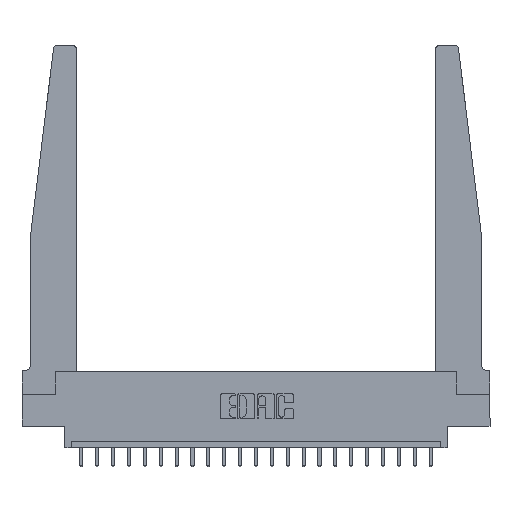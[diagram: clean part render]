
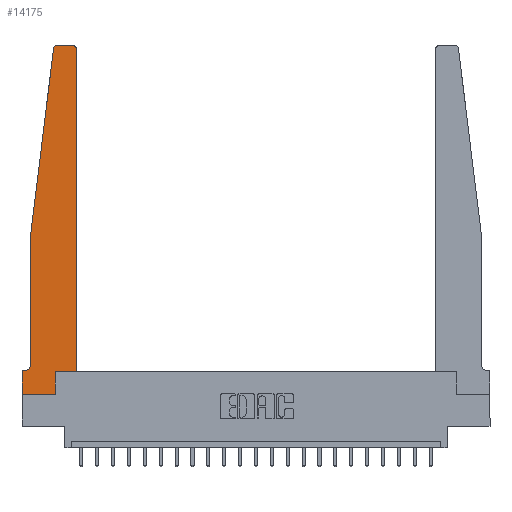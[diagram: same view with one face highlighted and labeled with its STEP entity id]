
A CAD part, top view. The second image highlights one B-rep face of the part: STEP entity #14175.
In plain terms, the highlighted planar face has unit normal (0, 0, 1).
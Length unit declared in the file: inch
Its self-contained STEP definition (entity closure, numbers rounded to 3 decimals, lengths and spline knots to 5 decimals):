
#63 = CARTESIAN_POINT ( 'NONE',  ( 0.425, 2.72, 0.37 ) ) ;
#163 = CARTESIAN_POINT ( 'NONE',  ( 0.065, 1.25, 0.37 ) ) ;
#206 = LINE ( 'NONE', #10738, #3052 ) ;
#305 = CARTESIAN_POINT ( 'NONE',  ( 0.2605, 0.18, 0.37 ) ) ;
#558 = EDGE_CURVE ( 'NONE', #3870, #2490, #2287, .T. ) ;
#1095 = EDGE_CURVE ( 'NONE', #10275, #9948, #206, .T. ) ;
#1131 = CARTESIAN_POINT ( 'NONE',  ( 0.25, 2.75, 0.37 ) ) ;
#1744 = VERTEX_POINT ( 'NONE', #19078 ) ;
#1785 = EDGE_CURVE ( 'NONE', #5472, #21026, #10588, .T. ) ;
#1889 = CARTESIAN_POINT ( 'NONE',  ( 0.27653, 2.75, 0.37 ) ) ;
#2123 = CARTESIAN_POINT ( 'NONE',  ( 0.2605, 0., 0.37 ) ) ;
#2154 = CARTESIAN_POINT ( 'NONE',  ( 0.065, 1.25, 0.37 ) ) ;
#2287 = CIRCLE ( 'NONE', #14850, 0.03 ) ;
#2384 = VERTEX_POINT ( 'NONE', #19950 ) ;
#2490 = VERTEX_POINT ( 'NONE', #11641 ) ;
#2630 = PLANE ( 'NONE',  #18287 ) ;
#2847 = LINE ( 'NONE', #16521, #13620 ) ;
#3021 = CARTESIAN_POINT ( 'NONE',  ( 0., 0., 0.37 ) ) ;
#3052 = VECTOR ( 'NONE', #17591, 39.37008 ) ;
#3132 = DIRECTION ( 'NONE',  ( 0., -1., 0. ) ) ;
#3254 = EDGE_CURVE ( 'NONE', #21026, #3870, #16509, .T. ) ;
#3502 = ORIENTED_EDGE ( 'NONE', *, *, #3254, .T. ) ;
#3577 = ORIENTED_EDGE ( 'NONE', *, *, #558, .T. ) ;
#3870 = VERTEX_POINT ( 'NONE', #1889 ) ;
#3942 = DIRECTION ( 'NONE',  ( 0., 0., -1. ) ) ;
#3983 = ORIENTED_EDGE ( 'NONE', *, *, #14107, .T. ) ;
#4412 = DIRECTION ( 'NONE',  ( 1., 0., 0. ) ) ;
#4774 = LINE ( 'NONE', #9807, #9773 ) ;
#4810 = LINE ( 'NONE', #3021, #7816 ) ;
#5472 = VERTEX_POINT ( 'NONE', #63 ) ;
#5702 = ORIENTED_EDGE ( 'NONE', *, *, #1785, .T. ) ;
#5886 = VECTOR ( 'NONE', #15826, 39.37008 ) ;
#6637 = CARTESIAN_POINT ( 'NONE',  ( 0.27653, 2.72, 0.37 ) ) ;
#6895 = LINE ( 'NONE', #163, #11553 ) ;
#7156 = ORIENTED_EDGE ( 'NONE', *, *, #13404, .T. ) ;
#7300 = ORIENTED_EDGE ( 'NONE', *, *, #17331, .T. ) ;
#7816 = VECTOR ( 'NONE', #3132, 39.37008 ) ;
#8459 = EDGE_CURVE ( 'NONE', #20569, #18451, #15411, .T. ) ;
#9541 = DIRECTION ( 'NONE',  ( -1., 0., 0. ) ) ;
#9643 = CARTESIAN_POINT ( 'NONE',  ( 0.065, 1.25, 0.37 ) ) ;
#9705 = CARTESIAN_POINT ( 'NONE',  ( 0.2605, 0.18, 0.37 ) ) ;
#9773 = VECTOR ( 'NONE', #18234, 39.37008 ) ;
#9807 = CARTESIAN_POINT ( 'NONE',  ( 0.065, 0.1875, 0.37 ) ) ;
#9948 = VERTEX_POINT ( 'NONE', #2123 ) ;
#10039 = AXIS2_PLACEMENT_3D ( 'NONE', #19746, #3942, #10870 ) ;
#10247 = EDGE_CURVE ( 'NONE', #2384, #10275, #4810, .T. ) ;
#10275 = VERTEX_POINT ( 'NONE', #20831 ) ;
#10371 = ORIENTED_EDGE ( 'NONE', *, *, #10247, .T. ) ;
#10466 = CARTESIAN_POINT ( 'NONE',  ( 0.065, 0.2375, 0.37 ) ) ;
#10588 = CIRCLE ( 'NONE', #19914, 0.03 ) ;
#10738 = CARTESIAN_POINT ( 'NONE',  ( 0., 0., 0.37 ) ) ;
#10870 = DIRECTION ( 'NONE',  ( -1., 0., 0. ) ) ;
#11105 = CARTESIAN_POINT ( 'NONE',  ( 0.395, 2.75, 0.37 ) ) ;
#11179 = DIRECTION ( 'NONE',  ( 1., 0., 0. ) ) ;
#11288 = CARTESIAN_POINT ( 'NONE',  ( 0.425, 0.18, 0.37 ) ) ;
#11553 = VECTOR ( 'NONE', #20481, 39.37008 ) ;
#11641 = CARTESIAN_POINT ( 'NONE',  ( 0.24675, 2.72367, 0.37 ) ) ;
#11917 = EDGE_CURVE ( 'NONE', #9948, #18796, #15677, .T. ) ;
#12160 = EDGE_LOOP ( 'NONE', ( #3502, #3577, #14645, #19969, #12771, #7300, #10371, #12710, #17135, #7156, #3983, #5702 ) ) ;
#12565 = DIRECTION ( 'NONE',  ( 1., 0., 0. ) ) ;
#12710 = ORIENTED_EDGE ( 'NONE', *, *, #1095, .T. ) ;
#12771 = ORIENTED_EDGE ( 'NONE', *, *, #8459, .T. ) ;
#13404 = EDGE_CURVE ( 'NONE', #18796, #1744, #20050, .T. ) ;
#13620 = VECTOR ( 'NONE', #19663, 39.37008 ) ;
#14107 = EDGE_CURVE ( 'NONE', #1744, #5472, #2847, .T. ) ;
#14175 = ADVANCED_FACE ( 'NONE', ( #16411 ), #2630, .T. ) ;
#14608 = CARTESIAN_POINT ( 'NONE',  ( 0., 0.1875, 0.37 ) ) ;
#14645 = ORIENTED_EDGE ( 'NONE', *, *, #20962, .T. ) ;
#14850 = AXIS2_PLACEMENT_3D ( 'NONE', #6637, #17510, #20994 ) ;
#15395 = VECTOR ( 'NONE', #11179, 39.37008 ) ;
#15411 = CIRCLE ( 'NONE', #10039, 0.05 ) ;
#15677 = LINE ( 'NONE', #305, #17836 ) ;
#15717 = DIRECTION ( 'NONE',  ( 0., 0., 1. ) ) ;
#15826 = DIRECTION ( 'NONE',  ( -0.122, -0.992, 0. ) ) ;
#16018 = VECTOR ( 'NONE', #9541, 39.37008 ) ;
#16411 = FACE_OUTER_BOUND ( 'NONE', #12160, .T. ) ;
#16509 = LINE ( 'NONE', #1131, #16018 ) ;
#16521 = CARTESIAN_POINT ( 'NONE',  ( 0.425, 0.18, 0.37 ) ) ;
#17049 = CARTESIAN_POINT ( 'NONE',  ( 0.015, 0.1875, 0.37 ) ) ;
#17135 = ORIENTED_EDGE ( 'NONE', *, *, #11917, .T. ) ;
#17331 = EDGE_CURVE ( 'NONE', #18451, #2384, #4774, .T. ) ;
#17510 = DIRECTION ( 'NONE',  ( 0., 0., 1. ) ) ;
#17517 = LINE ( 'NONE', #2154, #5886 ) ;
#17591 = DIRECTION ( 'NONE',  ( 1., 0., 0. ) ) ;
#17689 = DIRECTION ( 'NONE',  ( 0., 1., 0. ) ) ;
#17836 = VECTOR ( 'NONE', #17689, 39.37008 ) ;
#18234 = DIRECTION ( 'NONE',  ( -1., 0., 0. ) ) ;
#18287 = AXIS2_PLACEMENT_3D ( 'NONE', #14608, #19771, #4412 ) ;
#18345 = VERTEX_POINT ( 'NONE', #9643 ) ;
#18451 = VERTEX_POINT ( 'NONE', #17049 ) ;
#18796 = VERTEX_POINT ( 'NONE', #9705 ) ;
#18872 = EDGE_CURVE ( 'NONE', #18345, #20569, #6895, .T. ) ;
#19078 = CARTESIAN_POINT ( 'NONE',  ( 0.425, 0.18, 0.37 ) ) ;
#19663 = DIRECTION ( 'NONE',  ( 0., 1., 0. ) ) ;
#19746 = CARTESIAN_POINT ( 'NONE',  ( 0.015, 0.2375, 0.37 ) ) ;
#19771 = DIRECTION ( 'NONE',  ( 0., 0., 1. ) ) ;
#19914 = AXIS2_PLACEMENT_3D ( 'NONE', #21224, #15717, #12565 ) ;
#19950 = CARTESIAN_POINT ( 'NONE',  ( 0., 0.1875, 0.37 ) ) ;
#19969 = ORIENTED_EDGE ( 'NONE', *, *, #18872, .T. ) ;
#20050 = LINE ( 'NONE', #11288, #15395 ) ;
#20481 = DIRECTION ( 'NONE',  ( 0., -1., 0. ) ) ;
#20569 = VERTEX_POINT ( 'NONE', #10466 ) ;
#20831 = CARTESIAN_POINT ( 'NONE',  ( 0., 0., 0.37 ) ) ;
#20962 = EDGE_CURVE ( 'NONE', #2490, #18345, #17517, .T. ) ;
#20994 = DIRECTION ( 'NONE',  ( 1., 0., 0. ) ) ;
#21026 = VERTEX_POINT ( 'NONE', #11105 ) ;
#21224 = CARTESIAN_POINT ( 'NONE',  ( 0.395, 2.72, 0.37 ) ) ;
